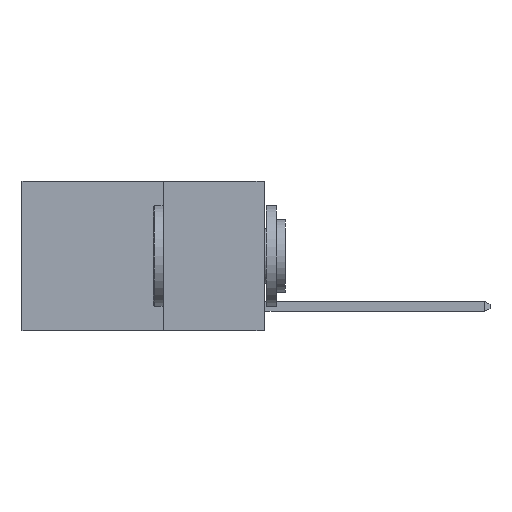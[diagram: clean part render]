
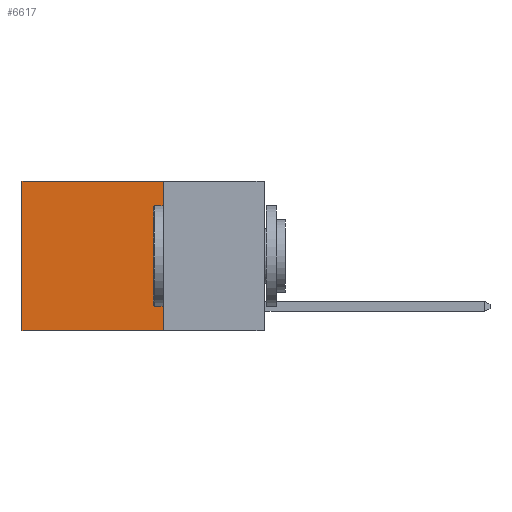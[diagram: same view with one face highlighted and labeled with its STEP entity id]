
A CAD part, left-side view. The second image highlights one B-rep face of the part: STEP entity #6617.
In plain terms, the highlighted planar face has unit normal (-1, 0, 0).
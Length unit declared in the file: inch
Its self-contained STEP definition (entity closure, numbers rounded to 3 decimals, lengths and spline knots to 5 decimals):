
#208 = EDGE_LOOP ( 'NONE', ( #6990, #1510, #7521, #9942 ) ) ;
#795 = VERTEX_POINT ( 'NONE', #3066 ) ;
#1510 = ORIENTED_EDGE ( 'NONE', *, *, #7853, .F. ) ;
#1563 = VECTOR ( 'NONE', #6731, 39.37008 ) ;
#2289 = CARTESIAN_POINT ( 'NONE',  ( 0.2625, 0.25, 0. ) ) ;
#2474 = CARTESIAN_POINT ( 'NONE',  ( 0.2625, 0.25, -0.37 ) ) ;
#2942 = CARTESIAN_POINT ( 'NONE',  ( 0.2625, 0.6, 0. ) ) ;
#2985 = VECTOR ( 'NONE', #3342, 39.37008 ) ;
#3066 = CARTESIAN_POINT ( 'NONE',  ( 0.2625, 0.25, -0.37 ) ) ;
#3342 = DIRECTION ( 'NONE',  ( 0., 1., 0. ) ) ;
#3352 = CARTESIAN_POINT ( 'NONE',  ( 0.2625, 0.25, 0. ) ) ;
#3612 = VERTEX_POINT ( 'NONE', #4673 ) ;
#3748 = DIRECTION ( 'NONE',  ( 0., 0., -1. ) ) ;
#4360 = VECTOR ( 'NONE', #8912, 39.37008 ) ;
#4544 = EDGE_CURVE ( 'NONE', #5614, #795, #8744, .T. ) ;
#4673 = CARTESIAN_POINT ( 'NONE',  ( 0.2625, 0.6, -0.37 ) ) ;
#5255 = VECTOR ( 'NONE', #5529, 39.37008 ) ;
#5277 = LINE ( 'NONE', #2474, #2985 ) ;
#5438 = FACE_OUTER_BOUND ( 'NONE', #208, .T. ) ;
#5529 = DIRECTION ( 'NONE',  ( 0., 0., -1. ) ) ;
#5614 = VERTEX_POINT ( 'NONE', #7348 ) ;
#6209 = PLANE ( 'NONE',  #9172 ) ;
#6617 = ADVANCED_FACE ( 'NONE', ( #5438 ), #6209, .F. ) ;
#6731 = DIRECTION ( 'NONE',  ( 0., 0., -1. ) ) ;
#6990 = ORIENTED_EDGE ( 'NONE', *, *, #8751, .T. ) ;
#7348 = CARTESIAN_POINT ( 'NONE',  ( 0.2625, 0.25, 0. ) ) ;
#7521 = ORIENTED_EDGE ( 'NONE', *, *, #4544, .F. ) ;
#7688 = EDGE_CURVE ( 'NONE', #5614, #9606, #8927, .T. ) ;
#7853 = EDGE_CURVE ( 'NONE', #795, #3612, #5277, .T. ) ;
#8641 = DIRECTION ( 'NONE',  ( 1., 0., 0. ) ) ;
#8744 = LINE ( 'NONE', #3352, #1563 ) ;
#8751 = EDGE_CURVE ( 'NONE', #9606, #3612, #9742, .T. ) ;
#8912 = DIRECTION ( 'NONE',  ( 0., 1., 0. ) ) ;
#8927 = LINE ( 'NONE', #2289, #4360 ) ;
#9172 = AXIS2_PLACEMENT_3D ( 'NONE', #10143, #8641, #3748 ) ;
#9606 = VERTEX_POINT ( 'NONE', #9750 ) ;
#9742 = LINE ( 'NONE', #2942, #5255 ) ;
#9750 = CARTESIAN_POINT ( 'NONE',  ( 0.2625, 0.6, 0. ) ) ;
#9942 = ORIENTED_EDGE ( 'NONE', *, *, #7688, .T. ) ;
#10143 = CARTESIAN_POINT ( 'NONE',  ( 0.2625, 0.25, 0. ) ) ;
